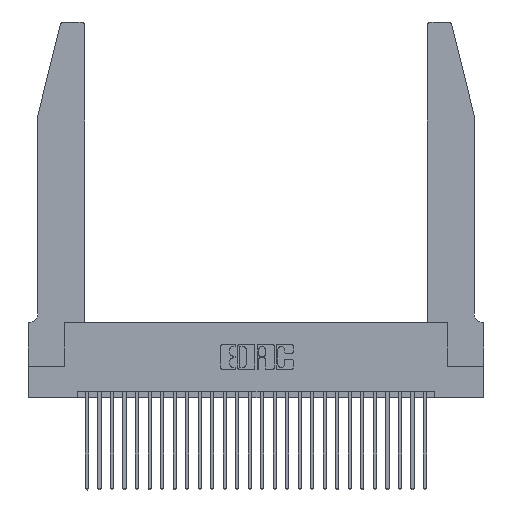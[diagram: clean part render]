
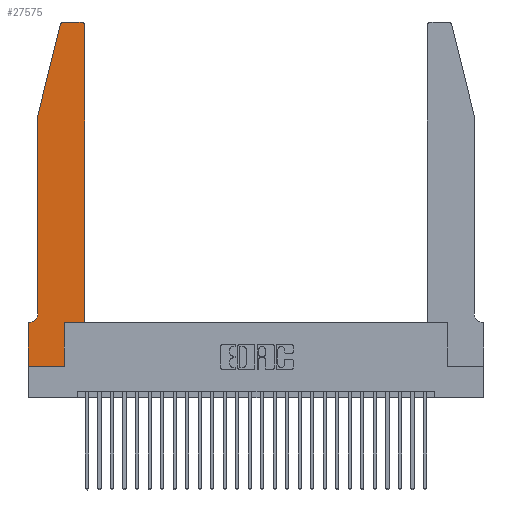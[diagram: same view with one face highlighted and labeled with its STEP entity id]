
A CAD part, top view. The second image highlights one B-rep face of the part: STEP entity #27575.
In plain terms, the highlighted planar face has unit normal (0, 0, 1).
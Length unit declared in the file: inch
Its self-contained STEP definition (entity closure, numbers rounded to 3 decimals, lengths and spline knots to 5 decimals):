
#31 = ORIENTED_EDGE ( 'NONE', *, *, #3894, .T. ) ;
#531 = VECTOR ( 'NONE', #7855, 39.37008 ) ;
#619 = VERTEX_POINT ( 'NONE', #7293 ) ;
#631 = ORIENTED_EDGE ( 'NONE', *, *, #19188, .T. ) ;
#1104 = ORIENTED_EDGE ( 'NONE', *, *, #23782, .T. ) ;
#1886 = CARTESIAN_POINT ( 'NONE',  ( 0.0755, 0.35, 0.37 ) ) ;
#2001 = ORIENTED_EDGE ( 'NONE', *, *, #24792, .T. ) ;
#2562 = CARTESIAN_POINT ( 'NONE',  ( 0.2865, 0., 0.37 ) ) ;
#3243 = CARTESIAN_POINT ( 'NONE',  ( 0.2865, 0.35, 0.37 ) ) ;
#3894 = EDGE_CURVE ( 'NONE', #12744, #7599, #16150, .T. ) ;
#4085 = CARTESIAN_POINT ( 'NONE',  ( 0., 0., 0.37 ) ) ;
#4329 = VECTOR ( 'NONE', #23588, 39.37008 ) ;
#4597 = EDGE_CURVE ( 'NONE', #7599, #28654, #12972, .T. ) ;
#5511 = VERTEX_POINT ( 'NONE', #3243 ) ;
#5659 = ORIENTED_EDGE ( 'NONE', *, *, #9570, .T. ) ;
#5725 = VECTOR ( 'NONE', #17424, 39.37008 ) ;
#5740 = CARTESIAN_POINT ( 'NONE',  ( 0.0055, 0.35, 0.37 ) ) ;
#6024 = ORIENTED_EDGE ( 'NONE', *, *, #16081, .T. ) ;
#6199 = VERTEX_POINT ( 'NONE', #18132 ) ;
#6263 = CARTESIAN_POINT ( 'NONE',  ( 0.2605, 2.75, 0.37 ) ) ;
#6311 = DIRECTION ( 'NONE',  ( 0., 0., 1. ) ) ;
#6765 = ORIENTED_EDGE ( 'NONE', *, *, #16238, .T. ) ;
#6969 = CARTESIAN_POINT ( 'NONE',  ( 0.0055, 0.42, 0.37 ) ) ;
#7098 = ORIENTED_EDGE ( 'NONE', *, *, #25613, .T. ) ;
#7154 = DIRECTION ( 'NONE',  ( 1., 0., 0. ) ) ;
#7257 = DIRECTION ( 'NONE',  ( 0., 0., 1. ) ) ;
#7293 = CARTESIAN_POINT ( 'NONE',  ( 0.0755, 0.42, 0.37 ) ) ;
#7599 = VERTEX_POINT ( 'NONE', #8075 ) ;
#7855 = DIRECTION ( 'NONE',  ( 0., -1., 0. ) ) ;
#7925 = CIRCLE ( 'NONE', #20850, 0.07 ) ;
#8075 = CARTESIAN_POINT ( 'NONE',  ( 0.4505, 2.72, 0.37 ) ) ;
#8135 = DIRECTION ( 'NONE',  ( -0.239, -0.971, 0. ) ) ;
#8145 = LINE ( 'NONE', #16928, #4329 ) ;
#8655 = LINE ( 'NONE', #6263, #16629 ) ;
#9472 = PLANE ( 'NONE',  #11729 ) ;
#9570 = EDGE_CURVE ( 'NONE', #5511, #12744, #17557, .T. ) ;
#10028 = LINE ( 'NONE', #4085, #28395 ) ;
#10053 = VERTEX_POINT ( 'NONE', #20340 ) ;
#11014 = VERTEX_POINT ( 'NONE', #24672 ) ;
#11239 = VERTEX_POINT ( 'NONE', #5740 ) ;
#11519 = DIRECTION ( 'NONE',  ( -1., 0., 0. ) ) ;
#11729 = AXIS2_PLACEMENT_3D ( 'NONE', #20278, #7257, #7154 ) ;
#11808 = DIRECTION ( 'NONE',  ( 1., 0., 0. ) ) ;
#12037 = CIRCLE ( 'NONE', #16532, 0.03 ) ;
#12358 = EDGE_CURVE ( 'NONE', #16111, #25645, #14629, .T. ) ;
#12502 = DIRECTION ( 'NONE',  ( 1., 0., 0. ) ) ;
#12744 = VERTEX_POINT ( 'NONE', #16373 ) ;
#12945 = ORIENTED_EDGE ( 'NONE', *, *, #12358, .T. ) ;
#12972 = CIRCLE ( 'NONE', #26249, 0.03 ) ;
#14600 = EDGE_CURVE ( 'NONE', #619, #11239, #7925, .T. ) ;
#14629 = LINE ( 'NONE', #27874, #15336 ) ;
#14989 = DIRECTION ( 'NONE',  ( -1., 0., 0. ) ) ;
#15223 = VECTOR ( 'NONE', #18185, 39.37008 ) ;
#15267 = ORIENTED_EDGE ( 'NONE', *, *, #15502, .T. ) ;
#15336 = VECTOR ( 'NONE', #8135, 39.37008 ) ;
#15502 = EDGE_CURVE ( 'NONE', #11014, #6199, #24071, .T. ) ;
#16081 = EDGE_CURVE ( 'NONE', #21206, #5511, #8145, .T. ) ;
#16105 = DIRECTION ( 'NONE',  ( 0., 0., -1. ) ) ;
#16111 = VERTEX_POINT ( 'NONE', #17024 ) ;
#16150 = LINE ( 'NONE', #28509, #16470 ) ;
#16238 = EDGE_CURVE ( 'NONE', #11239, #11014, #17534, .T. ) ;
#16246 = ORIENTED_EDGE ( 'NONE', *, *, #14600, .T. ) ;
#16290 = CARTESIAN_POINT ( 'NONE',  ( 0.0755, 2., 0.37 ) ) ;
#16373 = CARTESIAN_POINT ( 'NONE',  ( 0.4505, 0.35, 0.37 ) ) ;
#16470 = VECTOR ( 'NONE', #21495, 39.37008 ) ;
#16532 = AXIS2_PLACEMENT_3D ( 'NONE', #16649, #25436, #11808 ) ;
#16629 = VECTOR ( 'NONE', #14989, 39.37008 ) ;
#16649 = CARTESIAN_POINT ( 'NONE',  ( 0.284, 2.72, 0.37 ) ) ;
#16928 = CARTESIAN_POINT ( 'NONE',  ( 0.2865, 0.35, 0.37 ) ) ;
#17024 = CARTESIAN_POINT ( 'NONE',  ( 0.25487, 2.72718, 0.37 ) ) ;
#17150 = CARTESIAN_POINT ( 'NONE',  ( 0.4505, 0.35, 0.37 ) ) ;
#17267 = CARTESIAN_POINT ( 'NONE',  ( 0.4205, 2.72, 0.37 ) ) ;
#17424 = DIRECTION ( 'NONE',  ( -1., 0., 0. ) ) ;
#17534 = LINE ( 'NONE', #1886, #5725 ) ;
#17557 = LINE ( 'NONE', #17150, #22398 ) ;
#18132 = CARTESIAN_POINT ( 'NONE',  ( 0., 0., 0.37 ) ) ;
#18177 = CARTESIAN_POINT ( 'NONE',  ( 0.4205, 2.75, 0.37 ) ) ;
#18185 = DIRECTION ( 'NONE',  ( 0., -1., 0. ) ) ;
#19032 = LINE ( 'NONE', #20123, #15223 ) ;
#19188 = EDGE_CURVE ( 'NONE', #28654, #10053, #8655, .T. ) ;
#20123 = CARTESIAN_POINT ( 'NONE',  ( 0.0755, 2., 0.37 ) ) ;
#20278 = CARTESIAN_POINT ( 'NONE',  ( 0., 0.35, 0.37 ) ) ;
#20340 = CARTESIAN_POINT ( 'NONE',  ( 0.284, 2.75, 0.37 ) ) ;
#20850 = AXIS2_PLACEMENT_3D ( 'NONE', #6969, #16105, #11519 ) ;
#21206 = VERTEX_POINT ( 'NONE', #2562 ) ;
#21495 = DIRECTION ( 'NONE',  ( 0., 1., 0. ) ) ;
#22398 = VECTOR ( 'NONE', #12502, 39.37008 ) ;
#23588 = DIRECTION ( 'NONE',  ( 0., 1., 0. ) ) ;
#23627 = DIRECTION ( 'NONE',  ( 1., 0., 0. ) ) ;
#23782 = EDGE_CURVE ( 'NONE', #6199, #21206, #10028, .T. ) ;
#24071 = LINE ( 'NONE', #27688, #531 ) ;
#24672 = CARTESIAN_POINT ( 'NONE',  ( 0., 0.35, 0.37 ) ) ;
#24792 = EDGE_CURVE ( 'NONE', #25645, #619, #19032, .T. ) ;
#25421 = ORIENTED_EDGE ( 'NONE', *, *, #4597, .T. ) ;
#25436 = DIRECTION ( 'NONE',  ( 0., 0., 1. ) ) ;
#25613 = EDGE_CURVE ( 'NONE', #10053, #16111, #12037, .T. ) ;
#25645 = VERTEX_POINT ( 'NONE', #16290 ) ;
#25701 = EDGE_LOOP ( 'NONE', ( #631, #7098, #12945, #2001, #16246, #6765, #15267, #1104, #6024, #5659, #31, #25421 ) ) ;
#26118 = FACE_OUTER_BOUND ( 'NONE', #25701, .T. ) ;
#26249 = AXIS2_PLACEMENT_3D ( 'NONE', #17267, #6311, #23627 ) ;
#27575 = ADVANCED_FACE ( 'NONE', ( #26118 ), #9472, .T. ) ;
#27688 = CARTESIAN_POINT ( 'NONE',  ( 0., 0., 0.37 ) ) ;
#27874 = CARTESIAN_POINT ( 'NONE',  ( 0.0755, 2., 0.37 ) ) ;
#28395 = VECTOR ( 'NONE', #28557, 39.37008 ) ;
#28509 = CARTESIAN_POINT ( 'NONE',  ( 0.4505, 0.35, 0.37 ) ) ;
#28557 = DIRECTION ( 'NONE',  ( 1., 0., 0. ) ) ;
#28654 = VERTEX_POINT ( 'NONE', #18177 ) ;
